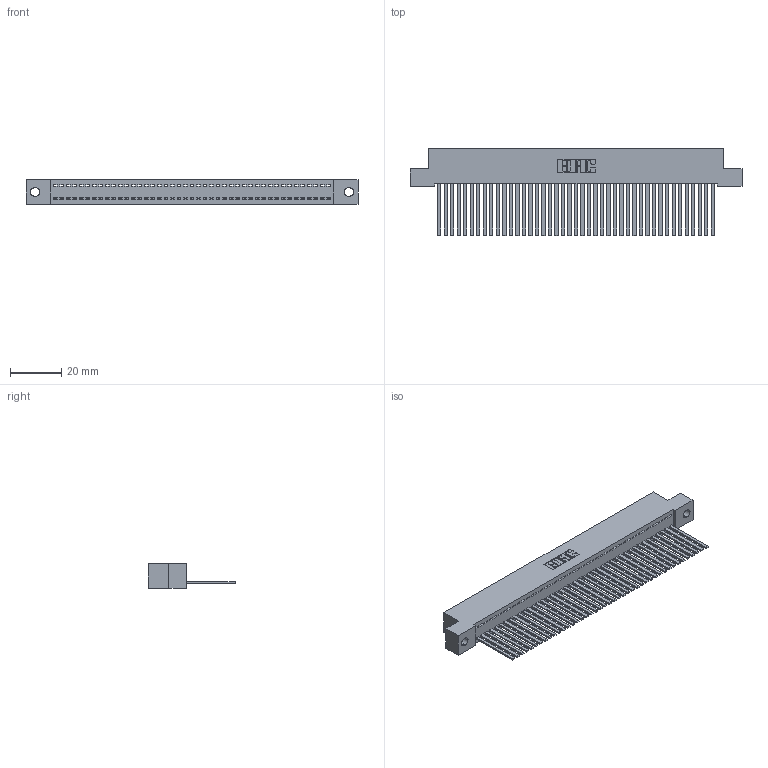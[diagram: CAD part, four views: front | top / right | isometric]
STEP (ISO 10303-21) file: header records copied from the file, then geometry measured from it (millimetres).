
FILE_DESCRIPTION (( 'STEP AP203' ), '1' );
FILE_NAME ('342-043-544-102.STEP', '2018-08-12T13:58:37', ( '' ), ( '' ), 'SwSTEP 2.0', 'SolidWorks 2016', '' );
FILE_SCHEMA (( 'CONFIG_CONTROL_DESIGN' ));
Length unit declared in the file: inch
Products named in the file (3): 342 Part_.128 Slot; 345-292-001_345-293-144; 342-043-544-102
Assembly tree (44 placements, depth 2):
  342-043-544-102
    342 Part_.128 Slot
    345-292-001_345-293-144  x43
Bounding box: 129.54 x 34.3 x 9.4 mm (x, y, z)
Volume: 11807.6 mm3; surface area: 18534.6 mm2
Topology: 44 solids, 44 shells, 2350 faces, 7105 edges, 4678 vertices
Faces by surface type: plane 1704, cylinder 646
Entity records: 25977 total; most frequent: CARTESIAN_POINT 4487, ORIENTED_EDGE 4466, DIRECTION 3779, EDGE_CURVE 2233, LINE 2109, VECTOR 2109, VERTEX_POINT 1486, AXIS2_PLACEMENT_3D 835
